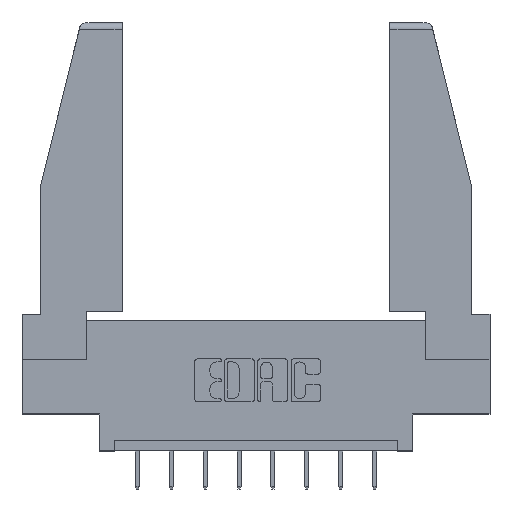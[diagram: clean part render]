
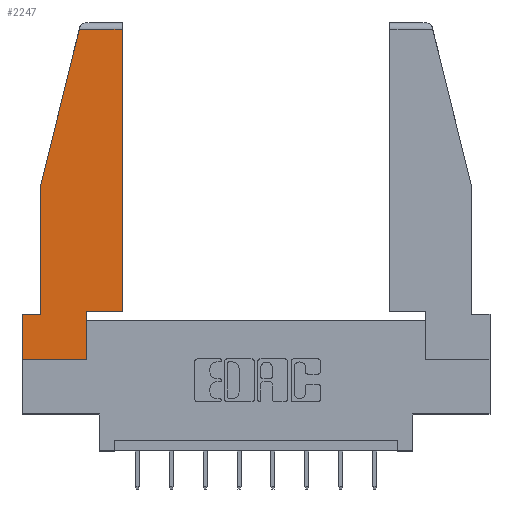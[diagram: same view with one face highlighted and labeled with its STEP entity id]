
A CAD part, top view. The second image highlights one B-rep face of the part: STEP entity #2247.
In plain terms, the highlighted planar face has unit normal (0, 0, 1).
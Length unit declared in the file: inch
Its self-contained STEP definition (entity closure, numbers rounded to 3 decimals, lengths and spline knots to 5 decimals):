
#371 = VERTEX_POINT ( 'NONE', #10363 ) ;
#455 = LINE ( 'NONE', #6389, #1364 ) ;
#557 = CARTESIAN_POINT ( 'NONE',  ( 0.086, 0.21, 0. ) ) ;
#561 = ORIENTED_EDGE ( 'NONE', *, *, #3395, .T. ) ;
#1112 = DIRECTION ( 'NONE',  ( 0., -1., 0. ) ) ;
#1316 = EDGE_CURVE ( 'NONE', #6547, #10857, #2669, .T. ) ;
#1347 = VECTOR ( 'NONE', #11279, 39.37008 ) ;
#1364 = VECTOR ( 'NONE', #3363, 39.37008 ) ;
#1541 = CARTESIAN_POINT ( 'NONE',  ( 0.297, 0., 0. ) ) ;
#1623 = ORIENTED_EDGE ( 'NONE', *, *, #8779, .T. ) ;
#1790 = ORIENTED_EDGE ( 'NONE', *, *, #1316, .T. ) ;
#2083 = ORIENTED_EDGE ( 'NONE', *, *, #12375, .T. ) ;
#2247 = ADVANCED_FACE ( 'NONE', ( #3412 ), #10821, .T. ) ;
#2577 = VECTOR ( 'NONE', #4299, 39.37008 ) ;
#2665 = CARTESIAN_POINT ( 'NONE',  ( 0., 0., 0. ) ) ;
#2669 = LINE ( 'NONE', #2665, #5673 ) ;
#2889 = LINE ( 'NONE', #8057, #2577 ) ;
#3149 = CARTESIAN_POINT ( 'NONE',  ( 0., 0.21, 0. ) ) ;
#3284 = DIRECTION ( 'NONE',  ( -1., 0., 0. ) ) ;
#3363 = DIRECTION ( 'NONE',  ( 0., 1., 0. ) ) ;
#3393 = VECTOR ( 'NONE', #1112, 39.37008 ) ;
#3395 = EDGE_CURVE ( 'NONE', #371, #6626, #2889, .T. ) ;
#3412 = FACE_OUTER_BOUND ( 'NONE', #12006, .T. ) ;
#3569 = ORIENTED_EDGE ( 'NONE', *, *, #5611, .T. ) ;
#3829 = CARTESIAN_POINT ( 'NONE',  ( 0., 0.21, 0. ) ) ;
#4026 = LINE ( 'NONE', #7128, #1347 ) ;
#4299 = DIRECTION ( 'NONE',  ( 0., 1., 0. ) ) ;
#4910 = AXIS2_PLACEMENT_3D ( 'NONE', #10861, #7950, #9841 ) ;
#5041 = CARTESIAN_POINT ( 'NONE',  ( 0., 0., 0. ) ) ;
#5115 = CARTESIAN_POINT ( 'NONE',  ( 0.2636, 1.52, 0. ) ) ;
#5546 = CARTESIAN_POINT ( 'NONE',  ( 0., 0.21, 0. ) ) ;
#5611 = EDGE_CURVE ( 'NONE', #6626, #12218, #10860, .T. ) ;
#5673 = VECTOR ( 'NONE', #9663, 39.37008 ) ;
#6101 = LINE ( 'NONE', #7122, #3393 ) ;
#6366 = CARTESIAN_POINT ( 'NONE',  ( 0.086, 0.8, 0. ) ) ;
#6389 = CARTESIAN_POINT ( 'NONE',  ( 0.297, 0., 0. ) ) ;
#6449 = LINE ( 'NONE', #5546, #11935 ) ;
#6488 = VECTOR ( 'NONE', #3284, 39.37008 ) ;
#6547 = VERTEX_POINT ( 'NONE', #5041 ) ;
#6564 = VERTEX_POINT ( 'NONE', #557 ) ;
#6626 = VERTEX_POINT ( 'NONE', #9273 ) ;
#6781 = VECTOR ( 'NONE', #7321, 39.37008 ) ;
#6833 = ORIENTED_EDGE ( 'NONE', *, *, #8923, .T. ) ;
#6890 = DIRECTION ( 'NONE',  ( 1., 0., 0. ) ) ;
#7122 = CARTESIAN_POINT ( 'NONE',  ( 0.086, 0.8, 0. ) ) ;
#7128 = CARTESIAN_POINT ( 'NONE',  ( 0.271, 1.55, 0. ) ) ;
#7294 = VECTOR ( 'NONE', #6890, 39.37008 ) ;
#7321 = DIRECTION ( 'NONE',  ( -1., 0., 0. ) ) ;
#7582 = DIRECTION ( 'NONE',  ( 0., -1., 0. ) ) ;
#7667 = ORIENTED_EDGE ( 'NONE', *, *, #9876, .T. ) ;
#7950 = DIRECTION ( 'NONE',  ( 0., 0., 1. ) ) ;
#8026 = VERTEX_POINT ( 'NONE', #11637 ) ;
#8057 = CARTESIAN_POINT ( 'NONE',  ( 0.461, 0.223, 0. ) ) ;
#8084 = VERTEX_POINT ( 'NONE', #3829 ) ;
#8321 = CARTESIAN_POINT ( 'NONE',  ( 0., 1.52, 0. ) ) ;
#8779 = EDGE_CURVE ( 'NONE', #10857, #8026, #455, .T. ) ;
#8923 = EDGE_CURVE ( 'NONE', #8084, #6547, #6449, .T. ) ;
#9267 = EDGE_CURVE ( 'NONE', #12218, #11807, #4026, .T. ) ;
#9273 = CARTESIAN_POINT ( 'NONE',  ( 0.461, 1.52, 0. ) ) ;
#9501 = ORIENTED_EDGE ( 'NONE', *, *, #12989, .T. ) ;
#9663 = DIRECTION ( 'NONE',  ( 1., 0., 0. ) ) ;
#9841 = DIRECTION ( 'NONE',  ( 1., 0., 0. ) ) ;
#9876 = EDGE_CURVE ( 'NONE', #11807, #6564, #6101, .T. ) ;
#10363 = CARTESIAN_POINT ( 'NONE',  ( 0.461, 0.223, 0. ) ) ;
#10489 = ORIENTED_EDGE ( 'NONE', *, *, #9267, .T. ) ;
#10594 = LINE ( 'NONE', #12844, #7294 ) ;
#10821 = PLANE ( 'NONE',  #4910 ) ;
#10857 = VERTEX_POINT ( 'NONE', #1541 ) ;
#10860 = LINE ( 'NONE', #8321, #6781 ) ;
#10861 = CARTESIAN_POINT ( 'NONE',  ( 0., 0., 0. ) ) ;
#11279 = DIRECTION ( 'NONE',  ( -0.239, -0.971, 0. ) ) ;
#11500 = LINE ( 'NONE', #3149, #6488 ) ;
#11637 = CARTESIAN_POINT ( 'NONE',  ( 0.297, 0.223, 0. ) ) ;
#11807 = VERTEX_POINT ( 'NONE', #6366 ) ;
#11935 = VECTOR ( 'NONE', #7582, 39.37008 ) ;
#12006 = EDGE_LOOP ( 'NONE', ( #561, #3569, #10489, #7667, #9501, #6833, #1790, #1623, #2083 ) ) ;
#12218 = VERTEX_POINT ( 'NONE', #5115 ) ;
#12375 = EDGE_CURVE ( 'NONE', #8026, #371, #10594, .T. ) ;
#12844 = CARTESIAN_POINT ( 'NONE',  ( 0.297, 0.223, 0. ) ) ;
#12989 = EDGE_CURVE ( 'NONE', #6564, #8084, #11500, .T. ) ;
